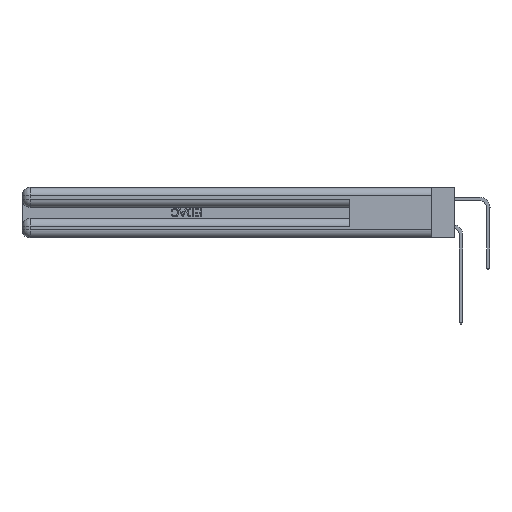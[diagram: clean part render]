
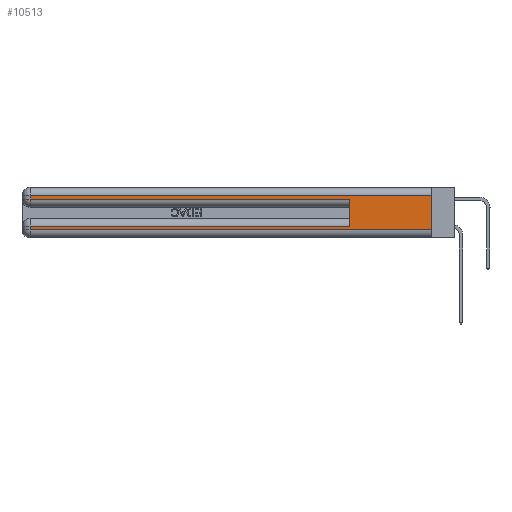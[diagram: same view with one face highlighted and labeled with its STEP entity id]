
A CAD part, left-side view. The second image highlights one B-rep face of the part: STEP entity #10513.
In plain terms, the highlighted planar face has unit normal (-1, 0, 0).
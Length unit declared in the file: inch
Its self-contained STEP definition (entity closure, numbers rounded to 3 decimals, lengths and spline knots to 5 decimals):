
#353 = VECTOR ( 'NONE', #38955, 39.37008 ) ;
#1114 = EDGE_CURVE ( 'NONE', #15233, #42685, #24377, .T. ) ;
#1246 = CARTESIAN_POINT ( 'NONE',  ( 0., 0., 0.37 ) ) ;
#6139 = VECTOR ( 'NONE', #23885, 39.37008 ) ;
#6552 = CARTESIAN_POINT ( 'NONE',  ( 0., 0., 0.31 ) ) ;
#6950 = DIRECTION ( 'NONE',  ( 0., 0., -1. ) ) ;
#7148 = VERTEX_POINT ( 'NONE', #15024 ) ;
#7281 = LINE ( 'NONE', #16220, #36340 ) ;
#8266 = EDGE_CURVE ( 'NONE', #28065, #42685, #26300, .T. ) ;
#9923 = EDGE_CURVE ( 'NONE', #7148, #26081, #34430, .T. ) ;
#10158 = ORIENTED_EDGE ( 'NONE', *, *, #8266, .T. ) ;
#10297 = ORIENTED_EDGE ( 'NONE', *, *, #34808, .T. ) ;
#10430 = EDGE_CURVE ( 'NONE', #13852, #28065, #23102, .T. ) ;
#10513 = ADVANCED_FACE ( 'NONE', ( #18311 ), #48578, .F. ) ;
#10745 = VERTEX_POINT ( 'NONE', #30800 ) ;
#10819 = CARTESIAN_POINT ( 'NONE',  ( 0., 0.6, 0.145 ) ) ;
#13068 = VECTOR ( 'NONE', #44969, 39.37008 ) ;
#13852 = VERTEX_POINT ( 'NONE', #23739 ) ;
#14037 = CARTESIAN_POINT ( 'NONE',  ( 0., 2.94, 0.37 ) ) ;
#15024 = CARTESIAN_POINT ( 'NONE',  ( 0., 0.6, 0.085 ) ) ;
#15233 = VERTEX_POINT ( 'NONE', #6552 ) ;
#16220 = CARTESIAN_POINT ( 'NONE',  ( 0., 0., 0.31 ) ) ;
#16227 = ORIENTED_EDGE ( 'NONE', *, *, #33518, .T. ) ;
#17831 = DIRECTION ( 'NONE',  ( 0., 0., -1. ) ) ;
#18274 = CARTESIAN_POINT ( 'NONE',  ( 0., 0., 0.285 ) ) ;
#18311 = FACE_OUTER_BOUND ( 'NONE', #42156, .T. ) ;
#19876 = DIRECTION ( 'NONE',  ( 0., 0., -1. ) ) ;
#20413 = LINE ( 'NONE', #46416, #353 ) ;
#20891 = VECTOR ( 'NONE', #22118, 39.37008 ) ;
#21967 = VECTOR ( 'NONE', #19876, 39.37008 ) ;
#22118 = DIRECTION ( 'NONE',  ( 0., -1., 0. ) ) ;
#23102 = LINE ( 'NONE', #14037, #42104 ) ;
#23739 = CARTESIAN_POINT ( 'NONE',  ( 0., 2.94, 0.085 ) ) ;
#23878 = DIRECTION ( 'NONE',  ( 0., 1., 0. ) ) ;
#23885 = DIRECTION ( 'NONE',  ( 0., -1., 0. ) ) ;
#24200 = VERTEX_POINT ( 'NONE', #40992 ) ;
#24377 = LINE ( 'NONE', #1246, #21967 ) ;
#25843 = CARTESIAN_POINT ( 'NONE',  ( 0., 0., 0.37 ) ) ;
#26081 = VERTEX_POINT ( 'NONE', #47007 ) ;
#26300 = LINE ( 'NONE', #42808, #6139 ) ;
#26378 = ORIENTED_EDGE ( 'NONE', *, *, #1114, .F. ) ;
#27262 = ORIENTED_EDGE ( 'NONE', *, *, #10430, .T. ) ;
#28065 = VERTEX_POINT ( 'NONE', #35739 ) ;
#29668 = DIRECTION ( 'NONE',  ( 1., 0., 0. ) ) ;
#30286 = AXIS2_PLACEMENT_3D ( 'NONE', #25843, #29668, #6950 ) ;
#30800 = CARTESIAN_POINT ( 'NONE',  ( 0., 2.94, 0.285 ) ) ;
#32664 = LINE ( 'NONE', #42753, #41588 ) ;
#32790 = ORIENTED_EDGE ( 'NONE', *, *, #9923, .F. ) ;
#33518 = EDGE_CURVE ( 'NONE', #7148, #13852, #20413, .T. ) ;
#34430 = LINE ( 'NONE', #10819, #13068 ) ;
#34808 = EDGE_CURVE ( 'NONE', #15233, #24200, #7281, .T. ) ;
#35739 = CARTESIAN_POINT ( 'NONE',  ( 0., 2.94, 0.06 ) ) ;
#36340 = VECTOR ( 'NONE', #23878, 39.37008 ) ;
#38955 = DIRECTION ( 'NONE',  ( 0., 1., 0. ) ) ;
#39187 = CARTESIAN_POINT ( 'NONE',  ( 0., 0., 0.06 ) ) ;
#40992 = CARTESIAN_POINT ( 'NONE',  ( 0., 2.94, 0.31 ) ) ;
#41024 = ORIENTED_EDGE ( 'NONE', *, *, #46881, .T. ) ;
#41588 = VECTOR ( 'NONE', #46575, 39.37008 ) ;
#42104 = VECTOR ( 'NONE', #17831, 39.37008 ) ;
#42156 = EDGE_LOOP ( 'NONE', ( #26378, #10297, #41024, #46426, #32790, #16227, #27262, #10158 ) ) ;
#42685 = VERTEX_POINT ( 'NONE', #39187 ) ;
#42753 = CARTESIAN_POINT ( 'NONE',  ( 0., 2.94, 0.37 ) ) ;
#42808 = CARTESIAN_POINT ( 'NONE',  ( 0., 0., 0.06 ) ) ;
#43465 = LINE ( 'NONE', #18274, #20891 ) ;
#44969 = DIRECTION ( 'NONE',  ( 0., 0., 1. ) ) ;
#45733 = EDGE_CURVE ( 'NONE', #10745, #26081, #43465, .T. ) ;
#46416 = CARTESIAN_POINT ( 'NONE',  ( 0., 0., 0.085 ) ) ;
#46426 = ORIENTED_EDGE ( 'NONE', *, *, #45733, .T. ) ;
#46575 = DIRECTION ( 'NONE',  ( 0., 0., -1. ) ) ;
#46881 = EDGE_CURVE ( 'NONE', #24200, #10745, #32664, .T. ) ;
#47007 = CARTESIAN_POINT ( 'NONE',  ( 0., 0.6, 0.285 ) ) ;
#48578 = PLANE ( 'NONE',  #30286 ) ;
